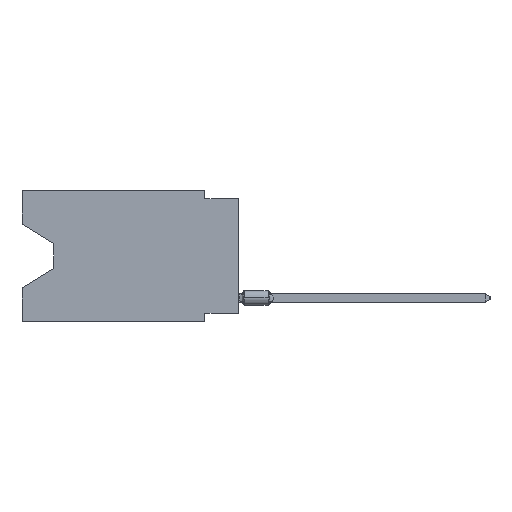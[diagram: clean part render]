
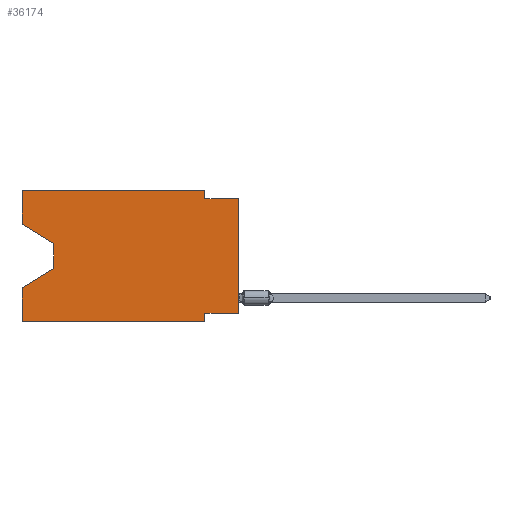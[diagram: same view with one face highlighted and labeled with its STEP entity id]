
A CAD part, left-side view. The second image highlights one B-rep face of the part: STEP entity #36174.
In plain terms, the highlighted planar face has unit normal (-1, 0, 0).
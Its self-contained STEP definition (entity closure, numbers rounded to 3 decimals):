
#109 = CARTESIAN_POINT ( 'NONE',  ( 0., 0., -9.271 ) ) ;
#249 = VERTEX_POINT ( 'NONE', #39965 ) ;
#390 = EDGE_CURVE ( 'NONE', #4192, #10406, #13447, .T. ) ;
#1690 = LINE ( 'NONE', #18611, #24023 ) ;
#1921 = ORIENTED_EDGE ( 'NONE', *, *, #30492, .T. ) ;
#2506 = LINE ( 'NONE', #32671, #20025 ) ;
#2634 = VERTEX_POINT ( 'NONE', #33100 ) ;
#3874 = EDGE_CURVE ( 'NONE', #10406, #21064, #6821, .T. ) ;
#4192 = VERTEX_POINT ( 'NONE', #20326 ) ;
#4296 = ORIENTED_EDGE ( 'NONE', *, *, #15899, .F. ) ;
#4880 = CARTESIAN_POINT ( 'NONE',  ( 0., 16.383, 0. ) ) ;
#5858 = LINE ( 'NONE', #28875, #39195 ) ;
#5922 = DIRECTION ( 'NONE',  ( 0., 0., 1. ) ) ;
#6821 = LINE ( 'NONE', #30493, #11710 ) ;
#7376 = EDGE_CURVE ( 'NONE', #26226, #2634, #31967, .T. ) ;
#8183 = EDGE_CURVE ( 'NONE', #21064, #15518, #2506, .T. ) ;
#8223 = VERTEX_POINT ( 'NONE', #23753 ) ;
#8501 = ORIENTED_EDGE ( 'NONE', *, *, #26514, .F. ) ;
#8804 = AXIS2_PLACEMENT_3D ( 'NONE', #4880, #25266, #14654 ) ;
#8860 = VECTOR ( 'NONE', #9365, 1000. ) ;
#9365 = DIRECTION ( 'NONE',  ( 0., 0., 1. ) ) ;
#9601 = ORIENTED_EDGE ( 'NONE', *, *, #7376, .T. ) ;
#9843 = ORIENTED_EDGE ( 'NONE', *, *, #18819, .F. ) ;
#9891 = EDGE_CURVE ( 'NONE', #38791, #22957, #40475, .T. ) ;
#10406 = VERTEX_POINT ( 'NONE', #36306 ) ;
#10585 = ORIENTED_EDGE ( 'NONE', *, *, #390, .T. ) ;
#10716 = CARTESIAN_POINT ( 'NONE',  ( 0., 2.54, -9.906 ) ) ;
#11710 = VECTOR ( 'NONE', #20069, 1000. ) ;
#12656 = CARTESIAN_POINT ( 'NONE',  ( 0., 16.383, 0. ) ) ;
#12820 = ORIENTED_EDGE ( 'NONE', *, *, #3874, .T. ) ;
#12980 = LINE ( 'NONE', #39487, #28209 ) ;
#13447 = LINE ( 'NONE', #23444, #25063 ) ;
#13752 = EDGE_CURVE ( 'NONE', #8223, #15518, #31771, .T. ) ;
#13829 = VECTOR ( 'NONE', #18626, 1000. ) ;
#14329 = ORIENTED_EDGE ( 'NONE', *, *, #35403, .F. ) ;
#14654 = DIRECTION ( 'NONE',  ( 0., 0., -1. ) ) ;
#15518 = VERTEX_POINT ( 'NONE', #27572 ) ;
#15899 = EDGE_CURVE ( 'NONE', #249, #42457, #12980, .T. ) ;
#15996 = CARTESIAN_POINT ( 'NONE',  ( 0., 2.54, -9.271 ) ) ;
#16360 = DIRECTION ( 'NONE',  ( 0., 0., -1. ) ) ;
#17006 = CARTESIAN_POINT ( 'NONE',  ( 0., 2.54, -9.906 ) ) ;
#18611 = CARTESIAN_POINT ( 'NONE',  ( 0., 2.54, 0. ) ) ;
#18626 = DIRECTION ( 'NONE',  ( 0., -1., 0. ) ) ;
#18819 = EDGE_CURVE ( 'NONE', #26226, #38791, #5858, .T. ) ;
#19622 = VECTOR ( 'NONE', #16360, 1000. ) ;
#20025 = VECTOR ( 'NONE', #22890, 1000. ) ;
#20069 = DIRECTION ( 'NONE',  ( 0., 0., -1. ) ) ;
#20286 = LINE ( 'NONE', #33539, #21917 ) ;
#20326 = CARTESIAN_POINT ( 'NONE',  ( 0., 16.383, -2.546 ) ) ;
#21064 = VERTEX_POINT ( 'NONE', #31214 ) ;
#21808 = FACE_OUTER_BOUND ( 'NONE', #22746, .T. ) ;
#21917 = VECTOR ( 'NONE', #30706, 1000. ) ;
#22223 = EDGE_CURVE ( 'NONE', #42457, #34015, #1690, .T. ) ;
#22746 = EDGE_LOOP ( 'NONE', ( #10585, #12820, #31334, #30260, #1921, #28360, #9843, #9601, #14329, #37422, #4296, #8501 ) ) ;
#22890 = DIRECTION ( 'NONE',  ( 0., 0.855, -0.519 ) ) ;
#22957 = VERTEX_POINT ( 'NONE', #10716 ) ;
#22975 = DIRECTION ( 'NONE',  ( 0., -1., 0. ) ) ;
#23444 = CARTESIAN_POINT ( 'NONE',  ( 0., 16.383, -2.546 ) ) ;
#23753 = CARTESIAN_POINT ( 'NONE',  ( 0., 16.383, -9.906 ) ) ;
#24023 = VECTOR ( 'NONE', #28389, 1000. ) ;
#25063 = VECTOR ( 'NONE', #36701, 1000. ) ;
#25112 = VECTOR ( 'NONE', #5922, 1000. ) ;
#25266 = DIRECTION ( 'NONE',  ( 1., 0., 0. ) ) ;
#26226 = VERTEX_POINT ( 'NONE', #109 ) ;
#26514 = EDGE_CURVE ( 'NONE', #4192, #249, #32823, .T. ) ;
#27572 = CARTESIAN_POINT ( 'NONE',  ( 0., 16.383, -7.36 ) ) ;
#28209 = VECTOR ( 'NONE', #22975, 1000. ) ;
#28360 = ORIENTED_EDGE ( 'NONE', *, *, #9891, .F. ) ;
#28389 = DIRECTION ( 'NONE',  ( 0., 0., -1. ) ) ;
#28618 = LINE ( 'NONE', #42100, #13829 ) ;
#28875 = CARTESIAN_POINT ( 'NONE',  ( 0., 0., -9.271 ) ) ;
#29594 = CARTESIAN_POINT ( 'NONE',  ( 0., 2.54, 0. ) ) ;
#29776 = DIRECTION ( 'NONE',  ( 0., 0., 1. ) ) ;
#30260 = ORIENTED_EDGE ( 'NONE', *, *, #13752, .F. ) ;
#30492 = EDGE_CURVE ( 'NONE', #8223, #22957, #28618, .T. ) ;
#30493 = CARTESIAN_POINT ( 'NONE',  ( 0., 13.97, -4.013 ) ) ;
#30706 = DIRECTION ( 'NONE',  ( 0., -1., 0. ) ) ;
#30927 = CARTESIAN_POINT ( 'NONE',  ( 0., 2.54, -0.635 ) ) ;
#31214 = CARTESIAN_POINT ( 'NONE',  ( 0., 13.97, -5.893 ) ) ;
#31334 = ORIENTED_EDGE ( 'NONE', *, *, #8183, .T. ) ;
#31771 = LINE ( 'NONE', #12656, #25112 ) ;
#31967 = LINE ( 'NONE', #35659, #8860 ) ;
#32671 = CARTESIAN_POINT ( 'NONE',  ( 0., 13.97, -5.893 ) ) ;
#32823 = LINE ( 'NONE', #36084, #39112 ) ;
#33100 = CARTESIAN_POINT ( 'NONE',  ( 0., 0., -0.635 ) ) ;
#33539 = CARTESIAN_POINT ( 'NONE',  ( 0., 0., -0.635 ) ) ;
#34015 = VERTEX_POINT ( 'NONE', #30927 ) ;
#35403 = EDGE_CURVE ( 'NONE', #34015, #2634, #20286, .T. ) ;
#35659 = CARTESIAN_POINT ( 'NONE',  ( 0., 0., 0. ) ) ;
#35815 = DIRECTION ( 'NONE',  ( 0., 1., 0. ) ) ;
#36084 = CARTESIAN_POINT ( 'NONE',  ( 0., 16.383, 0. ) ) ;
#36174 = ADVANCED_FACE ( 'NONE', ( #21808 ), #40951, .F. ) ;
#36306 = CARTESIAN_POINT ( 'NONE',  ( 0., 13.97, -4.013 ) ) ;
#36701 = DIRECTION ( 'NONE',  ( 0., -0.855, -0.519 ) ) ;
#37422 = ORIENTED_EDGE ( 'NONE', *, *, #22223, .F. ) ;
#38791 = VERTEX_POINT ( 'NONE', #15996 ) ;
#39112 = VECTOR ( 'NONE', #29776, 1000. ) ;
#39195 = VECTOR ( 'NONE', #35815, 1000. ) ;
#39487 = CARTESIAN_POINT ( 'NONE',  ( 0., 16.383, 0. ) ) ;
#39965 = CARTESIAN_POINT ( 'NONE',  ( 0., 16.383, 0. ) ) ;
#40475 = LINE ( 'NONE', #17006, #19622 ) ;
#40951 = PLANE ( 'NONE',  #8804 ) ;
#42100 = CARTESIAN_POINT ( 'NONE',  ( 0., 16.383, -9.906 ) ) ;
#42457 = VERTEX_POINT ( 'NONE', #29594 ) ;
